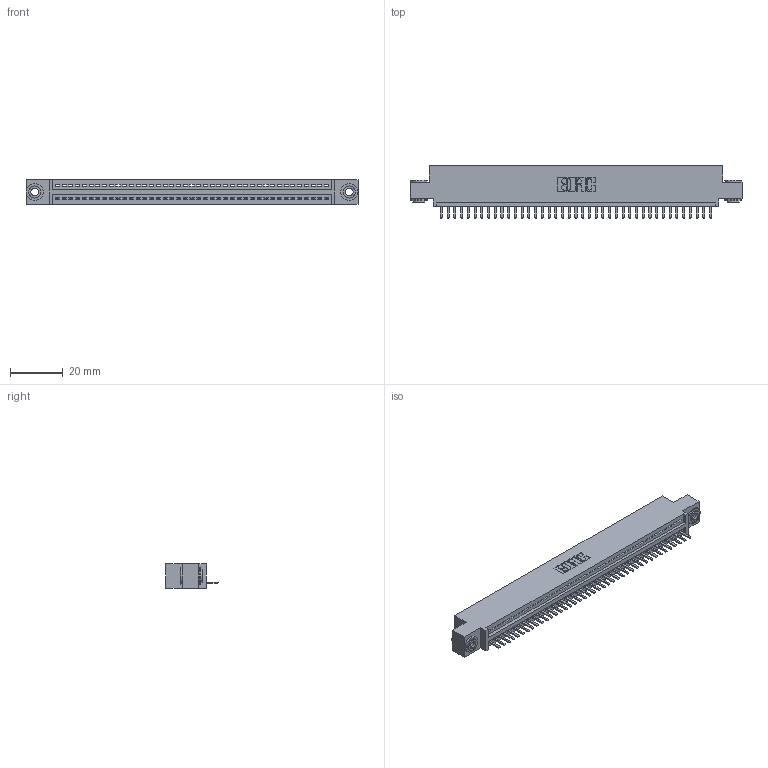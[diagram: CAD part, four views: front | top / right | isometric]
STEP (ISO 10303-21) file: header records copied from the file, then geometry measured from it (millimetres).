
FILE_DESCRIPTION (( 'STEP AP203' ), '1' );
FILE_NAME ('395-041-520-403.STEP', '2018-11-15T01:10:49', ( '' ), ( '' ), 'SwSTEP 2.0', 'SolidWorks 2016', '' );
FILE_SCHEMA (( 'CONFIG_CONTROL_DESIGN' ));
Length unit declared in the file: inch
Products named in the file (4): 395-041-520-403; 345 Part_0.110 Offset - 0.156 Dia-TH; 345-292-001_345-293-120; 345-250-002_345-250-002-102
Assembly tree (44 placements, depth 2):
  395-041-520-403
    345 Part_0.110 Offset - 0.156 Dia-TH
    345-292-001_345-293-120  x41
    345-250-002_345-250-002-102  x2
Bounding box: 125.35 x 19.68 x 9.4 mm (x, y, z)
Volume: 11725.7 mm3; surface area: 15479.3 mm2
Topology: 44 solids, 44 shells, 2710 faces, 7973 edges, 5202 vertices
Faces by surface type: plane 1816, cylinder 886, cone 8
Entity records: 31888 total; most frequent: CARTESIAN_POINT 5514, ORIENTED_EDGE 5470, DIRECTION 4835, EDGE_CURVE 2735, LINE 2411, VECTOR 2411, VERTEX_POINT 1818, AXIS2_PLACEMENT_3D 1212
